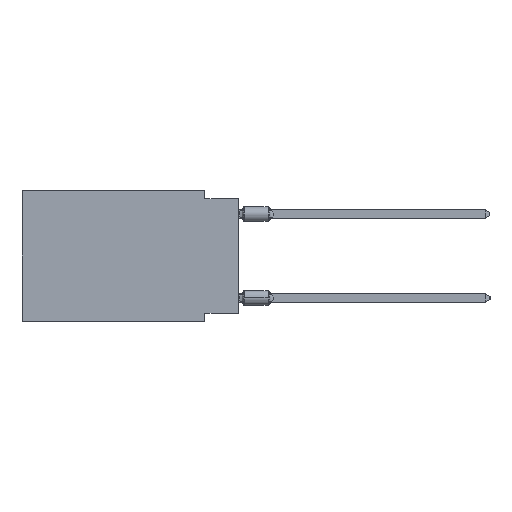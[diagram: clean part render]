
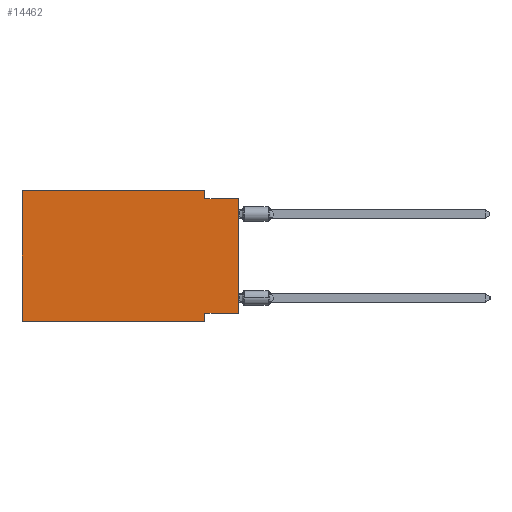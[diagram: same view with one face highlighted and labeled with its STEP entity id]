
A CAD part, left-side view. The second image highlights one B-rep face of the part: STEP entity #14462.
In plain terms, the highlighted planar face has unit normal (-1, 0, 0).
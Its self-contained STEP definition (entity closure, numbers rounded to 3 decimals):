
#1805 = PLANE ( 'NONE',  #58821 ) ;
#2113 = CARTESIAN_POINT ( 'NONE',  ( 0., 16.383, 0. ) ) ;
#2431 = ORIENTED_EDGE ( 'NONE', *, *, #50040, .T. ) ;
#2816 = VERTEX_POINT ( 'NONE', #62306 ) ;
#7173 = LINE ( 'NONE', #17416, #56662 ) ;
#7478 = CARTESIAN_POINT ( 'NONE',  ( 0., 0., 0. ) ) ;
#7714 = LINE ( 'NONE', #46882, #44167 ) ;
#8323 = VECTOR ( 'NONE', #33286, 1000. ) ;
#8776 = LINE ( 'NONE', #22886, #14167 ) ;
#8899 = ORIENTED_EDGE ( 'NONE', *, *, #60023, .F. ) ;
#9332 = CARTESIAN_POINT ( 'NONE',  ( 0., 0., -9.271 ) ) ;
#9366 = CARTESIAN_POINT ( 'NONE',  ( 0., 2.54, -9.906 ) ) ;
#9813 = EDGE_CURVE ( 'NONE', #20963, #60876, #39311, .T. ) ;
#9909 = VERTEX_POINT ( 'NONE', #15551 ) ;
#14167 = VECTOR ( 'NONE', #47624, 1000. ) ;
#14462 = ADVANCED_FACE ( 'NONE', ( #45768 ), #1805, .F. ) ;
#14759 = VERTEX_POINT ( 'NONE', #39289 ) ;
#15551 = CARTESIAN_POINT ( 'NONE',  ( 0., 0., -9.271 ) ) ;
#15868 = DIRECTION ( 'NONE',  ( 0., 0., 1. ) ) ;
#16795 = DIRECTION ( 'NONE',  ( 0., -1., 0. ) ) ;
#17196 = ORIENTED_EDGE ( 'NONE', *, *, #9813, .F. ) ;
#17416 = CARTESIAN_POINT ( 'NONE',  ( 0., 16.383, -9.906 ) ) ;
#19104 = ORIENTED_EDGE ( 'NONE', *, *, #24011, .F. ) ;
#20648 = VECTOR ( 'NONE', #15868, 1000. ) ;
#20963 = VERTEX_POINT ( 'NONE', #55093 ) ;
#21004 = CARTESIAN_POINT ( 'NONE',  ( 0., 2.54, -9.906 ) ) ;
#21373 = DIRECTION ( 'NONE',  ( 0., 0., -1. ) ) ;
#22886 = CARTESIAN_POINT ( 'NONE',  ( 0., 2.54, 0. ) ) ;
#23021 = ORIENTED_EDGE ( 'NONE', *, *, #42561, .F. ) ;
#24011 = EDGE_CURVE ( 'NONE', #14759, #54568, #57496, .T. ) ;
#24265 = CARTESIAN_POINT ( 'NONE',  ( 0., 2.54, -0.635 ) ) ;
#25503 = CARTESIAN_POINT ( 'NONE',  ( 0., 16.383, 0. ) ) ;
#26443 = EDGE_LOOP ( 'NONE', ( #32744, #8899, #23021, #40883, #17196, #2431, #19104, #55816 ) ) ;
#26572 = VERTEX_POINT ( 'NONE', #24265 ) ;
#28913 = VECTOR ( 'NONE', #62314, 1000. ) ;
#30329 = VERTEX_POINT ( 'NONE', #36204 ) ;
#30644 = VECTOR ( 'NONE', #59059, 1000. ) ;
#32744 = ORIENTED_EDGE ( 'NONE', *, *, #35331, .T. ) ;
#32963 = LINE ( 'NONE', #43258, #8323 ) ;
#33286 = DIRECTION ( 'NONE',  ( 0., -1., 0. ) ) ;
#35331 = EDGE_CURVE ( 'NONE', #9909, #2816, #51459, .T. ) ;
#36204 = CARTESIAN_POINT ( 'NONE',  ( 0., 2.54, 0. ) ) ;
#36452 = DIRECTION ( 'NONE',  ( 1., 0., 0. ) ) ;
#37241 = DIRECTION ( 'NONE',  ( 0., -1., 0. ) ) ;
#38086 = VECTOR ( 'NONE', #48539, 1000. ) ;
#39289 = CARTESIAN_POINT ( 'NONE',  ( 0., 2.54, -9.271 ) ) ;
#39311 = LINE ( 'NONE', #25503, #20648 ) ;
#40883 = ORIENTED_EDGE ( 'NONE', *, *, #59533, .F. ) ;
#42561 = EDGE_CURVE ( 'NONE', #30329, #26572, #8776, .T. ) ;
#43020 = EDGE_CURVE ( 'NONE', #9909, #14759, #53625, .T. ) ;
#43258 = CARTESIAN_POINT ( 'NONE',  ( 0., 0., -0.635 ) ) ;
#44167 = VECTOR ( 'NONE', #37241, 1000. ) ;
#45768 = FACE_OUTER_BOUND ( 'NONE', #26443, .T. ) ;
#46882 = CARTESIAN_POINT ( 'NONE',  ( 0., 16.383, 0. ) ) ;
#47624 = DIRECTION ( 'NONE',  ( 0., 0., -1. ) ) ;
#48539 = DIRECTION ( 'NONE',  ( 0., 0., -1. ) ) ;
#50040 = EDGE_CURVE ( 'NONE', #20963, #54568, #7173, .T. ) ;
#51459 = LINE ( 'NONE', #7478, #28913 ) ;
#53048 = CARTESIAN_POINT ( 'NONE',  ( 0., 16.383, 0. ) ) ;
#53625 = LINE ( 'NONE', #9332, #30644 ) ;
#54568 = VERTEX_POINT ( 'NONE', #21004 ) ;
#55093 = CARTESIAN_POINT ( 'NONE',  ( 0., 16.383, -9.906 ) ) ;
#55816 = ORIENTED_EDGE ( 'NONE', *, *, #43020, .F. ) ;
#56662 = VECTOR ( 'NONE', #16795, 1000. ) ;
#57496 = LINE ( 'NONE', #9366, #38086 ) ;
#58821 = AXIS2_PLACEMENT_3D ( 'NONE', #2113, #36452, #21373 ) ;
#59059 = DIRECTION ( 'NONE',  ( 0., 1., 0. ) ) ;
#59533 = EDGE_CURVE ( 'NONE', #60876, #30329, #7714, .T. ) ;
#60023 = EDGE_CURVE ( 'NONE', #26572, #2816, #32963, .T. ) ;
#60876 = VERTEX_POINT ( 'NONE', #53048 ) ;
#62306 = CARTESIAN_POINT ( 'NONE',  ( 0., 0., -0.635 ) ) ;
#62314 = DIRECTION ( 'NONE',  ( 0., 0., 1. ) ) ;
